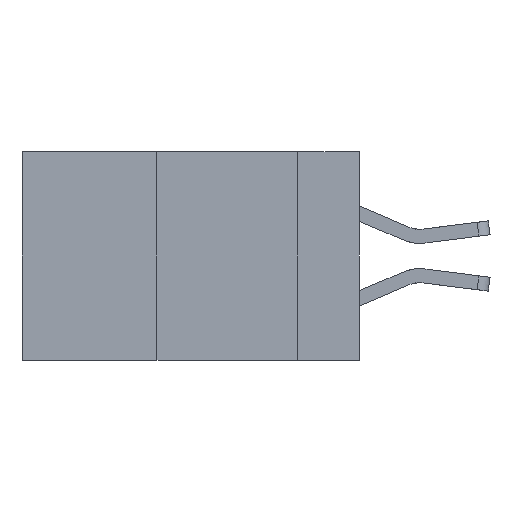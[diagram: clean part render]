
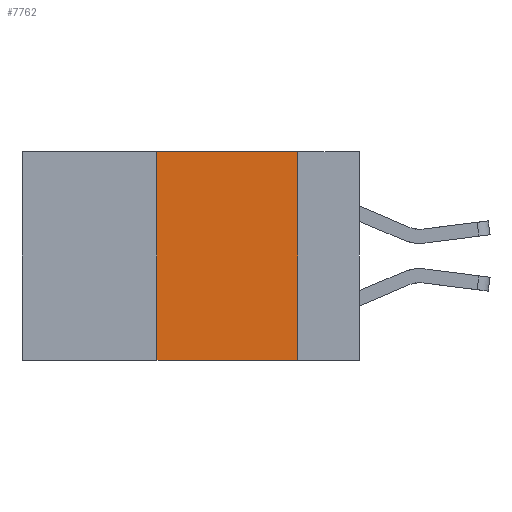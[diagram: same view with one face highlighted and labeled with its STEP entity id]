
A CAD part, left-side view. The second image highlights one B-rep face of the part: STEP entity #7762.
In plain terms, the highlighted planar face has unit normal (-1, 0, 0).
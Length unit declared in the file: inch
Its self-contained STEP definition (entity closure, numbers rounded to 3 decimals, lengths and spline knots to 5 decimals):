
#197 = LINE ( 'NONE', #1566, #6138 ) ;
#960 = EDGE_LOOP ( 'NONE', ( #6649, #7448, #5269, #7816 ) ) ;
#1380 = CARTESIAN_POINT ( 'NONE',  ( 0., 0.11, 0. ) ) ;
#1419 = LINE ( 'NONE', #4449, #6884 ) ;
#1487 = VERTEX_POINT ( 'NONE', #7987 ) ;
#1566 = CARTESIAN_POINT ( 'NONE',  ( 0., 0.6, 0. ) ) ;
#1637 = DIRECTION ( 'NONE',  ( 0., -1., 0. ) ) ;
#1738 = PLANE ( 'NONE',  #3891 ) ;
#1798 = CARTESIAN_POINT ( 'NONE',  ( 0., 0.36, 0. ) ) ;
#2465 = CARTESIAN_POINT ( 'NONE',  ( 0., 0.36, 0. ) ) ;
#2475 = LINE ( 'NONE', #2465, #7936 ) ;
#2760 = FACE_OUTER_BOUND ( 'NONE', #960, .T. ) ;
#2773 = CARTESIAN_POINT ( 'NONE',  ( 0., 0.6, -0.37 ) ) ;
#2922 = EDGE_CURVE ( 'NONE', #8067, #3272, #2475, .T. ) ;
#3112 = EDGE_CURVE ( 'NONE', #3272, #3838, #197, .T. ) ;
#3272 = VERTEX_POINT ( 'NONE', #1798 ) ;
#3838 = VERTEX_POINT ( 'NONE', #1380 ) ;
#3891 = AXIS2_PLACEMENT_3D ( 'NONE', #7262, #8716, #6431 ) ;
#4449 = CARTESIAN_POINT ( 'NONE',  ( 0., 0.11, 0. ) ) ;
#5269 = ORIENTED_EDGE ( 'NONE', *, *, #2922, .F. ) ;
#5282 = DIRECTION ( 'NONE',  ( 0., 0., -1. ) ) ;
#5593 = DIRECTION ( 'NONE',  ( 0., 0., 1. ) ) ;
#6138 = VECTOR ( 'NONE', #1637, 39.37008 ) ;
#6431 = DIRECTION ( 'NONE',  ( 0., 0., -1. ) ) ;
#6649 = ORIENTED_EDGE ( 'NONE', *, *, #9476, .F. ) ;
#6884 = VECTOR ( 'NONE', #5282, 39.37008 ) ;
#7020 = CARTESIAN_POINT ( 'NONE',  ( 0., 0.36, -0.37 ) ) ;
#7262 = CARTESIAN_POINT ( 'NONE',  ( 0., 0.6, 0. ) ) ;
#7448 = ORIENTED_EDGE ( 'NONE', *, *, #3112, .F. ) ;
#7459 = DIRECTION ( 'NONE',  ( 0., -1., 0. ) ) ;
#7762 = ADVANCED_FACE ( 'NONE', ( #2760 ), #1738, .F. ) ;
#7816 = ORIENTED_EDGE ( 'NONE', *, *, #8076, .T. ) ;
#7936 = VECTOR ( 'NONE', #5593, 39.37008 ) ;
#7987 = CARTESIAN_POINT ( 'NONE',  ( 0., 0.11, -0.37 ) ) ;
#8067 = VERTEX_POINT ( 'NONE', #7020 ) ;
#8076 = EDGE_CURVE ( 'NONE', #8067, #1487, #9056, .T. ) ;
#8716 = DIRECTION ( 'NONE',  ( 1., 0., 0. ) ) ;
#9056 = LINE ( 'NONE', #2773, #9553 ) ;
#9476 = EDGE_CURVE ( 'NONE', #3838, #1487, #1419, .T. ) ;
#9553 = VECTOR ( 'NONE', #7459, 39.37008 ) ;
